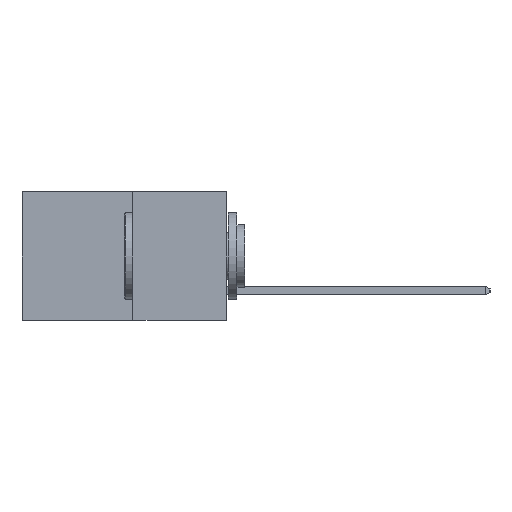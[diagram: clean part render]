
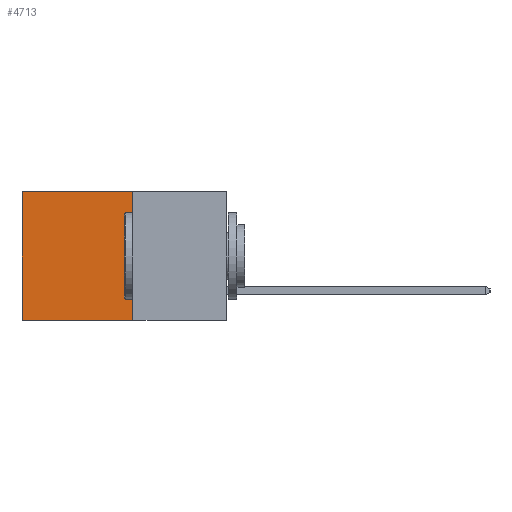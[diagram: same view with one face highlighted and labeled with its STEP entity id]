
A CAD part, left-side view. The second image highlights one B-rep face of the part: STEP entity #4713.
In plain terms, the highlighted planar face has unit normal (-1, 0, 0).
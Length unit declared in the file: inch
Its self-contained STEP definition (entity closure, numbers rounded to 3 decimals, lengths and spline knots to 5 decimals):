
#1163 = VECTOR ( 'NONE', #9704, 39.37008 ) ;
#1578 = ORIENTED_EDGE ( 'NONE', *, *, #2046, .T. ) ;
#1926 = CARTESIAN_POINT ( 'NONE',  ( 0.277, 0.59, -0.37 ) ) ;
#2046 = EDGE_CURVE ( 'NONE', #8826, #6381, #7471, .T. ) ;
#2405 = ORIENTED_EDGE ( 'NONE', *, *, #5996, .F. ) ;
#3129 = PLANE ( 'NONE',  #7607 ) ;
#3253 = DIRECTION ( 'NONE',  ( 0., 0., -1. ) ) ;
#3287 = DIRECTION ( 'NONE',  ( 1., 0., 0. ) ) ;
#4098 = CARTESIAN_POINT ( 'NONE',  ( 0.277, 0.27, -0.37 ) ) ;
#4494 = EDGE_CURVE ( 'NONE', #15017, #6381, #4593, .T. ) ;
#4593 = LINE ( 'NONE', #9752, #1163 ) ;
#4713 = ADVANCED_FACE ( 'NONE', ( #11074 ), #3129, .F. ) ;
#4716 = VECTOR ( 'NONE', #5498, 39.37008 ) ;
#5123 = LINE ( 'NONE', #5890, #4716 ) ;
#5293 = VERTEX_POINT ( 'NONE', #12578 ) ;
#5498 = DIRECTION ( 'NONE',  ( 0., 0., -1. ) ) ;
#5890 = CARTESIAN_POINT ( 'NONE',  ( 0.277, 0.27, -0.37 ) ) ;
#5996 = EDGE_CURVE ( 'NONE', #5293, #15017, #5123, .T. ) ;
#6381 = VERTEX_POINT ( 'NONE', #1926 ) ;
#6575 = EDGE_CURVE ( 'NONE', #5293, #8826, #10231, .T. ) ;
#6899 = VECTOR ( 'NONE', #13038, 39.37008 ) ;
#7471 = LINE ( 'NONE', #14007, #13649 ) ;
#7607 = AXIS2_PLACEMENT_3D ( 'NONE', #4098, #3287, #3253 ) ;
#7674 = CARTESIAN_POINT ( 'NONE',  ( 0.277, 0.59, 0. ) ) ;
#7681 = CARTESIAN_POINT ( 'NONE',  ( 0.277, 0.27, -0.37 ) ) ;
#8826 = VERTEX_POINT ( 'NONE', #7674 ) ;
#9704 = DIRECTION ( 'NONE',  ( 0., 1., 0. ) ) ;
#9752 = CARTESIAN_POINT ( 'NONE',  ( 0.277, 0.27, -0.37 ) ) ;
#10231 = LINE ( 'NONE', #13072, #6899 ) ;
#11074 = FACE_OUTER_BOUND ( 'NONE', #15126, .T. ) ;
#12578 = CARTESIAN_POINT ( 'NONE',  ( 0.277, 0.27, 0. ) ) ;
#13038 = DIRECTION ( 'NONE',  ( 0., 1., 0. ) ) ;
#13072 = CARTESIAN_POINT ( 'NONE',  ( 0.277, 0.27, 0. ) ) ;
#13649 = VECTOR ( 'NONE', #13883, 39.37008 ) ;
#13883 = DIRECTION ( 'NONE',  ( 0., 0., -1. ) ) ;
#14007 = CARTESIAN_POINT ( 'NONE',  ( 0.277, 0.59, -0.37 ) ) ;
#14869 = ORIENTED_EDGE ( 'NONE', *, *, #4494, .F. ) ;
#15017 = VERTEX_POINT ( 'NONE', #7681 ) ;
#15126 = EDGE_LOOP ( 'NONE', ( #1578, #14869, #2405, #15608 ) ) ;
#15608 = ORIENTED_EDGE ( 'NONE', *, *, #6575, .T. ) ;
